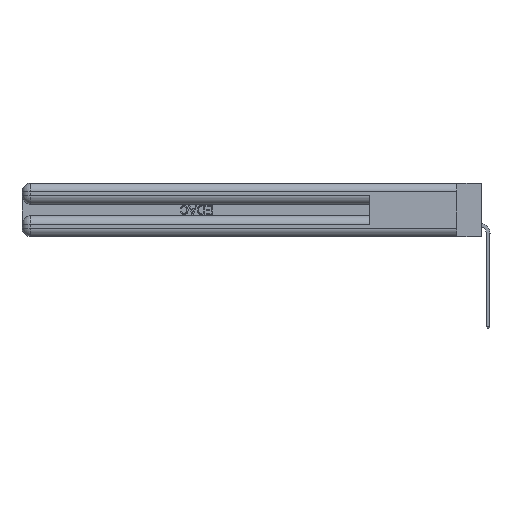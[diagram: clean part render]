
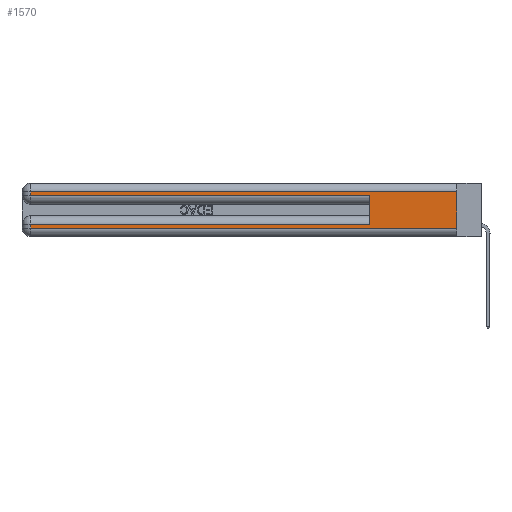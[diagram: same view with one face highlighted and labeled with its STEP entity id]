
A CAD part, left-side view. The second image highlights one B-rep face of the part: STEP entity #1570.
In plain terms, the highlighted planar face has unit normal (-1, 0, 0).
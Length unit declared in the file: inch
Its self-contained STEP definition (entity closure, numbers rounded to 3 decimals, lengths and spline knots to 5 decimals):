
#1506 = VERTEX_POINT ( 'NONE', #22692 ) ;
#1570 = ADVANCED_FACE ( 'NONE', ( #5317 ), #2715, .F. ) ;
#2389 = VERTEX_POINT ( 'NONE', #32902 ) ;
#2714 = ORIENTED_EDGE ( 'NONE', *, *, #7528, .T. ) ;
#2715 = PLANE ( 'NONE',  #37908 ) ;
#2981 = CARTESIAN_POINT ( 'NONE',  ( 0., 0.6, 0.145 ) ) ;
#3083 = DIRECTION ( 'NONE',  ( 0., 1., 0. ) ) ;
#4910 = LINE ( 'NONE', #29922, #37951 ) ;
#5317 = FACE_OUTER_BOUND ( 'NONE', #7314, .T. ) ;
#5767 = DIRECTION ( 'NONE',  ( 0., 0., -1. ) ) ;
#5969 = VECTOR ( 'NONE', #43557, 39.37008 ) ;
#6485 = VERTEX_POINT ( 'NONE', #23221 ) ;
#7314 = EDGE_LOOP ( 'NONE', ( #10869, #9868, #37392, #45954, #14070, #2714, #29111, #44918 ) ) ;
#7528 = EDGE_CURVE ( 'NONE', #11132, #20090, #39000, .T. ) ;
#8422 = DIRECTION ( 'NONE',  ( 0., 1., 0. ) ) ;
#9868 = ORIENTED_EDGE ( 'NONE', *, *, #25792, .T. ) ;
#10310 = LINE ( 'NONE', #10451, #43729 ) ;
#10451 = CARTESIAN_POINT ( 'NONE',  ( 0., 0., 0.06 ) ) ;
#10869 = ORIENTED_EDGE ( 'NONE', *, *, #12539, .F. ) ;
#11132 = VERTEX_POINT ( 'NONE', #45292 ) ;
#12243 = DIRECTION ( 'NONE',  ( 0., -1., 0. ) ) ;
#12539 = EDGE_CURVE ( 'NONE', #6485, #42933, #30874, .T. ) ;
#12677 = EDGE_CURVE ( 'NONE', #16367, #42933, #10310, .T. ) ;
#13400 = EDGE_CURVE ( 'NONE', #33314, #2389, #21826, .T. ) ;
#14070 = ORIENTED_EDGE ( 'NONE', *, *, #24771, .F. ) ;
#15607 = LINE ( 'NONE', #2981, #24069 ) ;
#16367 = VERTEX_POINT ( 'NONE', #37497 ) ;
#16521 = LINE ( 'NONE', #43408, #5969 ) ;
#16822 = VECTOR ( 'NONE', #12243, 39.37008 ) ;
#17360 = CARTESIAN_POINT ( 'NONE',  ( 0., 0., 0.06 ) ) ;
#17409 = DIRECTION ( 'NONE',  ( 0., -1., 0. ) ) ;
#18984 = VECTOR ( 'NONE', #44346, 39.37008 ) ;
#19186 = CARTESIAN_POINT ( 'NONE',  ( 0., 2.94, 0.37 ) ) ;
#20041 = DIRECTION ( 'NONE',  ( 0., 0., -1. ) ) ;
#20090 = VERTEX_POINT ( 'NONE', #34895 ) ;
#20500 = DIRECTION ( 'NONE',  ( 1., 0., 0. ) ) ;
#20611 = DIRECTION ( 'NONE',  ( 0., 0., 1. ) ) ;
#21826 = LINE ( 'NONE', #40951, #16822 ) ;
#22692 = CARTESIAN_POINT ( 'NONE',  ( 0., 2.94, 0.31 ) ) ;
#23221 = CARTESIAN_POINT ( 'NONE',  ( 0., 0., 0.31 ) ) ;
#24069 = VECTOR ( 'NONE', #20611, 39.37008 ) ;
#24343 = CARTESIAN_POINT ( 'NONE',  ( 0., 0., 0.085 ) ) ;
#24771 = EDGE_CURVE ( 'NONE', #11132, #2389, #15607, .T. ) ;
#25792 = EDGE_CURVE ( 'NONE', #6485, #1506, #4910, .T. ) ;
#26164 = CARTESIAN_POINT ( 'NONE',  ( 0., 2.94, 0.285 ) ) ;
#27946 = LINE ( 'NONE', #19186, #18984 ) ;
#29111 = ORIENTED_EDGE ( 'NONE', *, *, #36801, .T. ) ;
#29922 = CARTESIAN_POINT ( 'NONE',  ( 0., 0., 0.31 ) ) ;
#30874 = LINE ( 'NONE', #45125, #42688 ) ;
#32902 = CARTESIAN_POINT ( 'NONE',  ( 0., 0.6, 0.285 ) ) ;
#33314 = VERTEX_POINT ( 'NONE', #26164 ) ;
#34426 = CARTESIAN_POINT ( 'NONE',  ( 0., 0., 0.37 ) ) ;
#34895 = CARTESIAN_POINT ( 'NONE',  ( 0., 2.94, 0.085 ) ) ;
#36801 = EDGE_CURVE ( 'NONE', #20090, #16367, #16521, .T. ) ;
#37257 = VECTOR ( 'NONE', #3083, 39.37008 ) ;
#37392 = ORIENTED_EDGE ( 'NONE', *, *, #40165, .T. ) ;
#37497 = CARTESIAN_POINT ( 'NONE',  ( 0., 2.94, 0.06 ) ) ;
#37908 = AXIS2_PLACEMENT_3D ( 'NONE', #34426, #20500, #20041 ) ;
#37951 = VECTOR ( 'NONE', #8422, 39.37008 ) ;
#39000 = LINE ( 'NONE', #24343, #37257 ) ;
#40165 = EDGE_CURVE ( 'NONE', #1506, #33314, #27946, .T. ) ;
#40951 = CARTESIAN_POINT ( 'NONE',  ( 0., 0., 0.285 ) ) ;
#42688 = VECTOR ( 'NONE', #5767, 39.37008 ) ;
#42933 = VERTEX_POINT ( 'NONE', #17360 ) ;
#43408 = CARTESIAN_POINT ( 'NONE',  ( 0., 2.94, 0.37 ) ) ;
#43557 = DIRECTION ( 'NONE',  ( 0., 0., -1. ) ) ;
#43729 = VECTOR ( 'NONE', #17409, 39.37008 ) ;
#44346 = DIRECTION ( 'NONE',  ( 0., 0., -1. ) ) ;
#44918 = ORIENTED_EDGE ( 'NONE', *, *, #12677, .T. ) ;
#45125 = CARTESIAN_POINT ( 'NONE',  ( 0., 0., 0.37 ) ) ;
#45292 = CARTESIAN_POINT ( 'NONE',  ( 0., 0.6, 0.085 ) ) ;
#45954 = ORIENTED_EDGE ( 'NONE', *, *, #13400, .T. ) ;
